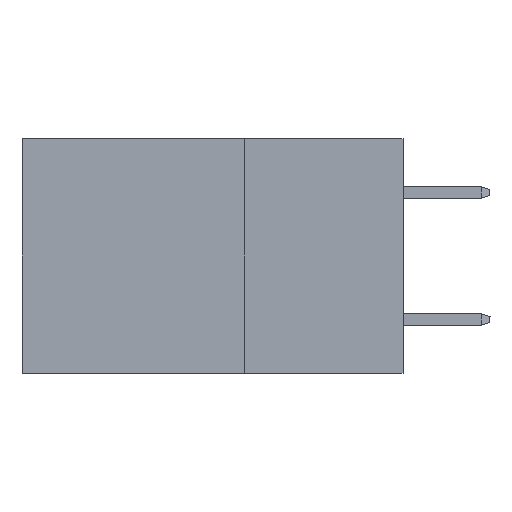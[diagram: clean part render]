
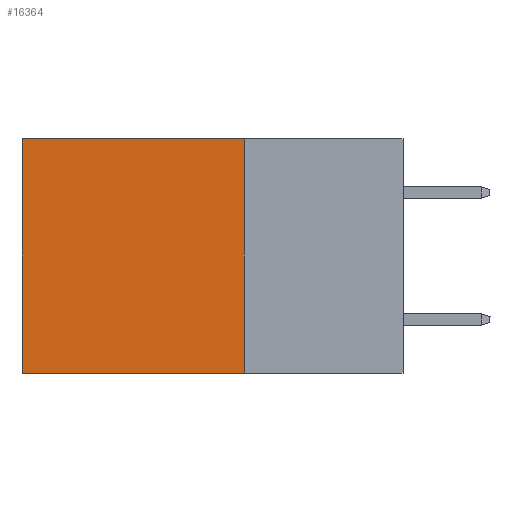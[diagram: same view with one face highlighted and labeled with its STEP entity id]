
A CAD part, left-side view. The second image highlights one B-rep face of the part: STEP entity #16364.
In plain terms, the highlighted planar face has unit normal (-1, 0, 0).
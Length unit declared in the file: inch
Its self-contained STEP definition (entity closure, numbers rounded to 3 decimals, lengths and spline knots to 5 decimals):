
#294 = LINE ( 'NONE', #13969, #20750 ) ;
#1399 = CARTESIAN_POINT ( 'NONE',  ( 0.2875, 0.25, 0. ) ) ;
#2690 = VERTEX_POINT ( 'NONE', #18120 ) ;
#4570 = VERTEX_POINT ( 'NONE', #12357 ) ;
#4815 = CARTESIAN_POINT ( 'NONE',  ( 0.2875, 0.25, 0. ) ) ;
#7128 = DIRECTION ( 'NONE',  ( 1., 0., 0. ) ) ;
#8474 = VECTOR ( 'NONE', #18670, 39.37008 ) ;
#8758 = EDGE_CURVE ( 'NONE', #11086, #10506, #21478, .T. ) ;
#9692 = CARTESIAN_POINT ( 'NONE',  ( 0.2875, 0.25, -0.37 ) ) ;
#10506 = VERTEX_POINT ( 'NONE', #22443 ) ;
#10786 = AXIS2_PLACEMENT_3D ( 'NONE', #4815, #7128, #11683 ) ;
#11086 = VERTEX_POINT ( 'NONE', #20329 ) ;
#11393 = PLANE ( 'NONE',  #10786 ) ;
#11683 = DIRECTION ( 'NONE',  ( 0., 0., -1. ) ) ;
#11883 = DIRECTION ( 'NONE',  ( 0., 0., -1. ) ) ;
#12031 = DIRECTION ( 'NONE',  ( 0., 0., -1. ) ) ;
#12357 = CARTESIAN_POINT ( 'NONE',  ( 0.2875, 0.6, -0.37 ) ) ;
#13099 = VECTOR ( 'NONE', #23588, 39.37008 ) ;
#13763 = FACE_OUTER_BOUND ( 'NONE', #19071, .T. ) ;
#13969 = CARTESIAN_POINT ( 'NONE',  ( 0.2875, 0.6, 0. ) ) ;
#14567 = LINE ( 'NONE', #9692, #8474 ) ;
#14579 = ORIENTED_EDGE ( 'NONE', *, *, #8758, .F. ) ;
#15365 = EDGE_CURVE ( 'NONE', #11086, #2690, #28418, .T. ) ;
#16364 = ADVANCED_FACE ( 'NONE', ( #13763 ), #11393, .F. ) ;
#16757 = CARTESIAN_POINT ( 'NONE',  ( 0.2875, 0.25, 0. ) ) ;
#17487 = ORIENTED_EDGE ( 'NONE', *, *, #15365, .T. ) ;
#18120 = CARTESIAN_POINT ( 'NONE',  ( 0.2875, 0.6, 0. ) ) ;
#18670 = DIRECTION ( 'NONE',  ( 0., 1., 0. ) ) ;
#19015 = EDGE_CURVE ( 'NONE', #10506, #4570, #14567, .T. ) ;
#19071 = EDGE_LOOP ( 'NONE', ( #25153, #19298, #14579, #17487 ) ) ;
#19298 = ORIENTED_EDGE ( 'NONE', *, *, #19015, .F. ) ;
#19457 = VECTOR ( 'NONE', #12031, 39.37008 ) ;
#20329 = CARTESIAN_POINT ( 'NONE',  ( 0.2875, 0.25, 0. ) ) ;
#20750 = VECTOR ( 'NONE', #11883, 39.37008 ) ;
#21478 = LINE ( 'NONE', #16757, #19457 ) ;
#22443 = CARTESIAN_POINT ( 'NONE',  ( 0.2875, 0.25, -0.37 ) ) ;
#23588 = DIRECTION ( 'NONE',  ( 0., 1., 0. ) ) ;
#24222 = EDGE_CURVE ( 'NONE', #2690, #4570, #294, .T. ) ;
#25153 = ORIENTED_EDGE ( 'NONE', *, *, #24222, .T. ) ;
#28418 = LINE ( 'NONE', #1399, #13099 ) ;
